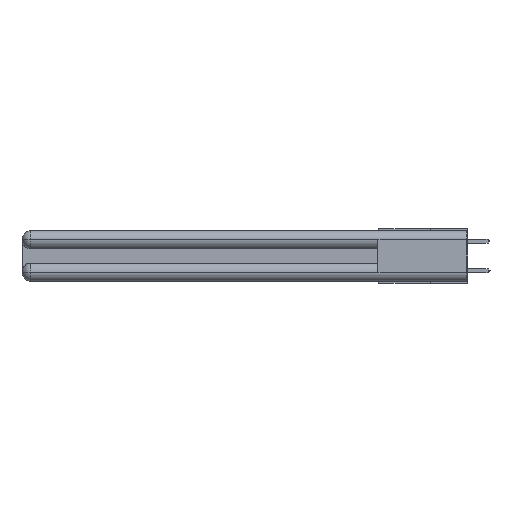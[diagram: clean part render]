
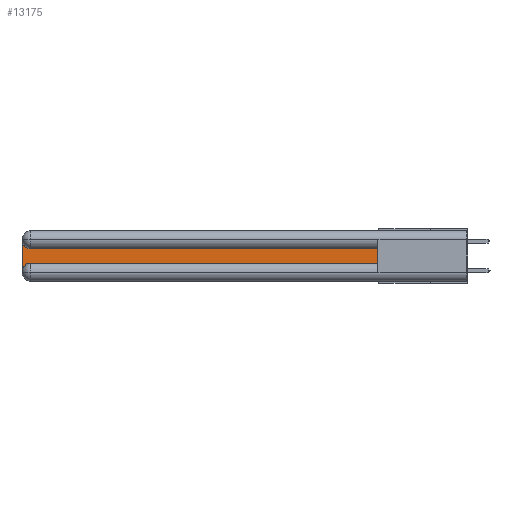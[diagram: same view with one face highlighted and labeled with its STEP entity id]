
A CAD part, left-side view. The second image highlights one B-rep face of the part: STEP entity #13175.
In plain terms, the highlighted planar face has unit normal (-1, 0, 0).
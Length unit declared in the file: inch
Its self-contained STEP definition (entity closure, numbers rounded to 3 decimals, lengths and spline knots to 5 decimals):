
#289 = CARTESIAN_POINT ( 'NONE',  ( 0.075, 3., -0.2175 ) ) ;
#1654 = ORIENTED_EDGE ( 'NONE', *, *, #3508, .T. ) ;
#1812 = VERTEX_POINT ( 'NONE', #18605 ) ;
#2212 = LINE ( 'NONE', #19190, #26834 ) ;
#2660 = DIRECTION ( 'NONE',  ( 0., 0., -1. ) ) ;
#3245 = CARTESIAN_POINT ( 'NONE',  ( 0.075, 2.94, -0.2175 ) ) ;
#3508 = EDGE_CURVE ( 'NONE', #21346, #26545, #23238, .T. ) ;
#4182 = EDGE_CURVE ( 'NONE', #26545, #5723, #21590, .T. ) ;
#4948 = ORIENTED_EDGE ( 'NONE', *, *, #17241, .T. ) ;
#5077 = DIRECTION ( 'NONE',  ( 1., 0., 0. ) ) ;
#5723 = VERTEX_POINT ( 'NONE', #14970 ) ;
#5756 = AXIS2_PLACEMENT_3D ( 'NONE', #14569, #18840, #14301 ) ;
#6490 = DIRECTION ( 'NONE',  ( 0., 0., 1. ) ) ;
#7203 = ORIENTED_EDGE ( 'NONE', *, *, #4182, .T. ) ;
#7237 = DIRECTION ( 'NONE',  ( 0., 0., -1. ) ) ;
#8033 = AXIS2_PLACEMENT_3D ( 'NONE', #16593, #22681, #12112 ) ;
#8620 = LINE ( 'NONE', #24876, #9273 ) ;
#9273 = VECTOR ( 'NONE', #10479, 39.37008 ) ;
#9493 = CARTESIAN_POINT ( 'NONE',  ( 0.075, 2.94, -0.1225 ) ) ;
#9572 = LINE ( 'NONE', #10599, #17021 ) ;
#9803 = CIRCLE ( 'NONE', #8033, 0.06 ) ;
#9895 = EDGE_CURVE ( 'NONE', #20498, #21346, #2212, .T. ) ;
#10479 = DIRECTION ( 'NONE',  ( 0., -1., 0. ) ) ;
#10599 = CARTESIAN_POINT ( 'NONE',  ( 0.075, 0.6, -0.2175 ) ) ;
#11972 = FACE_OUTER_BOUND ( 'NONE', #22293, .T. ) ;
#12112 = DIRECTION ( 'NONE',  ( 0., 0., -1. ) ) ;
#13175 = ADVANCED_FACE ( 'NONE', ( #11972 ), #20672, .F. ) ;
#14301 = DIRECTION ( 'NONE',  ( 0., 0., -1. ) ) ;
#14510 = EDGE_CURVE ( 'NONE', #23687, #1812, #8620, .T. ) ;
#14569 = CARTESIAN_POINT ( 'NONE',  ( 0.075, 3., -0.1225 ) ) ;
#14775 = ORIENTED_EDGE ( 'NONE', *, *, #15500, .T. ) ;
#14970 = CARTESIAN_POINT ( 'NONE',  ( 0.075, 3., -0.2775 ) ) ;
#15500 = EDGE_CURVE ( 'NONE', #1812, #20498, #9572, .T. ) ;
#16593 = CARTESIAN_POINT ( 'NONE',  ( 0.075, 2.94, -0.2775 ) ) ;
#17021 = VECTOR ( 'NONE', #6490, 39.37008 ) ;
#17241 = EDGE_CURVE ( 'NONE', #5723, #23687, #9803, .T. ) ;
#17723 = CARTESIAN_POINT ( 'NONE',  ( 0.075, 3., -0.0625 ) ) ;
#17791 = CARTESIAN_POINT ( 'NONE',  ( 0.075, 0.6, -0.1225 ) ) ;
#18605 = CARTESIAN_POINT ( 'NONE',  ( 0.075, 0.6, -0.2175 ) ) ;
#18840 = DIRECTION ( 'NONE',  ( 1., 0., 0. ) ) ;
#19190 = CARTESIAN_POINT ( 'NONE',  ( 0.075, 0.6, -0.1225 ) ) ;
#19308 = VECTOR ( 'NONE', #2660, 39.37008 ) ;
#19662 = CARTESIAN_POINT ( 'NONE',  ( 0.075, 2.94, -0.0625 ) ) ;
#20498 = VERTEX_POINT ( 'NONE', #17791 ) ;
#20672 = PLANE ( 'NONE',  #5756 ) ;
#21205 = ORIENTED_EDGE ( 'NONE', *, *, #9895, .T. ) ;
#21346 = VERTEX_POINT ( 'NONE', #9493 ) ;
#21590 = LINE ( 'NONE', #289, #19308 ) ;
#22293 = EDGE_LOOP ( 'NONE', ( #21205, #1654, #7203, #4948, #23726, #14775 ) ) ;
#22681 = DIRECTION ( 'NONE',  ( 1., 0., 0. ) ) ;
#22996 = DIRECTION ( 'NONE',  ( 0., 1., 0. ) ) ;
#23238 = CIRCLE ( 'NONE', #23474, 0.06 ) ;
#23474 = AXIS2_PLACEMENT_3D ( 'NONE', #19662, #5077, #7237 ) ;
#23687 = VERTEX_POINT ( 'NONE', #3245 ) ;
#23726 = ORIENTED_EDGE ( 'NONE', *, *, #14510, .T. ) ;
#24876 = CARTESIAN_POINT ( 'NONE',  ( 0.075, 0.6, -0.2175 ) ) ;
#26545 = VERTEX_POINT ( 'NONE', #17723 ) ;
#26834 = VECTOR ( 'NONE', #22996, 39.37008 ) ;
